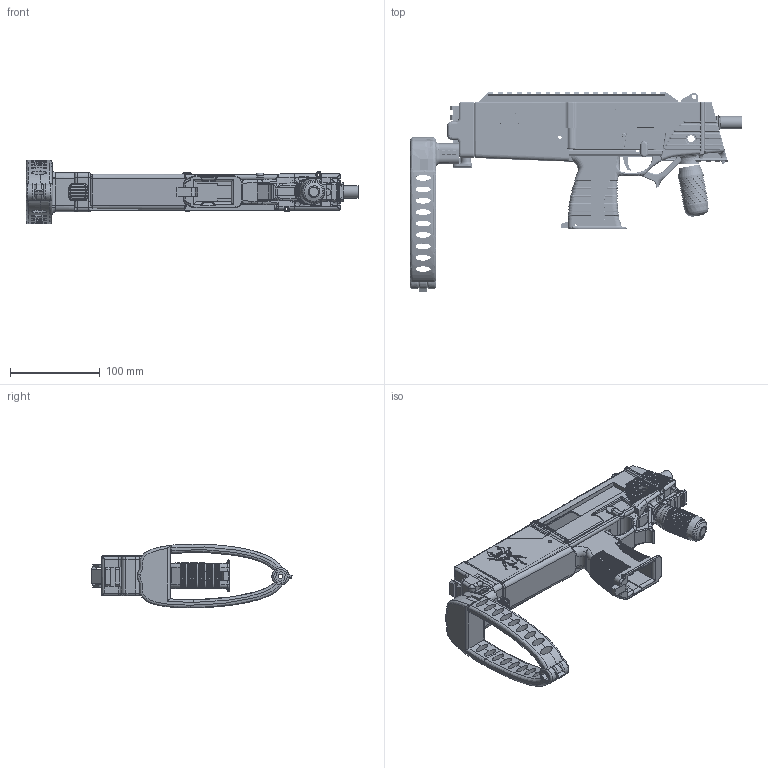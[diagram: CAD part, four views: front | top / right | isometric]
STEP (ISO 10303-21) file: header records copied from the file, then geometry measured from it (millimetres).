
FILE_DESCRIPTION(/* description */ (''),/* implementation_level */ '2;1');
FILE_NAME(/* name */ 'STL''s/Final Scarab Stuff/Scarab Master.step',/* time_stamp */ '2022-05-07T23:48:14-04:00',/* author */ (''),/* organization */ (''),/* preprocessor_version */ 'ST-DEVELOPER v18.1',/* originating_system */ 'Autodesk Translation Framework v10.14.0.1471',/* authorisation */ '');
FILE_SCHEMA (('AUTOMOTIVE_DESIGN { 1 0 10303 214 3 1 1 }'));
Products named in the file (9): Scarab MP7 Style; Upper Receiver v6; Trigger v2; Safety v3; Hammer v1; Sear_Bar v2; Trigger_Bar v1; Trigger_Pin v1; MagCatch v1
Assembly tree (8 placements, depth 2):
  Scarab MP7 Style
    Upper Receiver v6
    Trigger v2
    Safety v3
    Hammer v1
    Sear_Bar v2
    Trigger_Bar v1
    Trigger_Pin v1
    MagCatch v1
Bounding box: 370.15 x 223.7 x 71.14 mm (x, y, z)
Volume: 533867 mm3; surface area: 692065.5 mm2
Topology: 30 solids, 34 shells, 9909 faces, 25910 edges, 16102 vertices
Faces by surface type: plane 3583, cylinder 2842, bspline 2186, torus 1244, cone 47, sphere 7
Full cylindrical faces by diameter (mm): 3 x12, 3.073 x24, 3.175 x8, 3.4 x4, 3.429 x2, 3.5 x8, 4.039 x1, 4.089 x8, 4.572 x2, 4.65 x6, 4.699 x1, 4.7 x22, 4.75 x4, 4.757 x4, 4.9 x6, 5 x7, 5.08 x2, 5.461 x2, 5.5 x8, 5.588 x1, 5.65 x4, 5.69 x1, 5.7 x7, 5.893 x2, 6.096 x4, 6.2 x4, 6.35 x4, 6.477 x1, 6.604 x3, 7.239 x2
Entity records: 736761 total; most frequent: CARTESIAN_POINT 506966, ORIENTED_EDGE 51672, DIRECTION 43600, EDGE_CURVE 25836, VERTEX_POINT 16102, AXIS2_PLACEMENT_3D 16023, LINE 11554, VECTOR 11554
